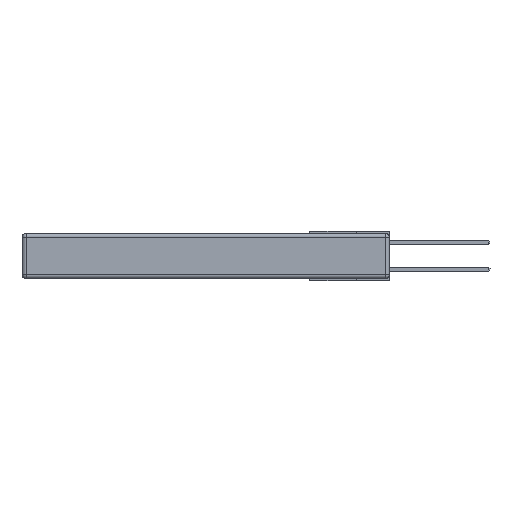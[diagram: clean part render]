
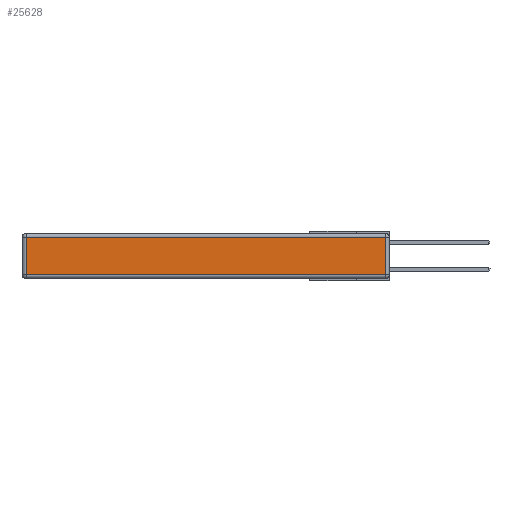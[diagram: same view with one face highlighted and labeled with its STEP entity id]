
A CAD part, left-side view. The second image highlights one B-rep face of the part: STEP entity #25628.
In plain terms, the highlighted planar face has unit normal (-1, 0, 0).
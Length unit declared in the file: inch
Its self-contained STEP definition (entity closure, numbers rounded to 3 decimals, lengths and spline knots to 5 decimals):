
#993 = VERTEX_POINT ( 'NONE', #25898 ) ;
#1000 = CARTESIAN_POINT ( 'NONE',  ( 0., 0.03, -0.03 ) ) ;
#3266 = VECTOR ( 'NONE', #28624, 39.37008 ) ;
#3453 = EDGE_CURVE ( 'NONE', #15135, #5135, #9915, .T. ) ;
#4842 = CARTESIAN_POINT ( 'NONE',  ( 0., 0.03, -0.343 ) ) ;
#5065 = LINE ( 'NONE', #4842, #3266 ) ;
#5135 = VERTEX_POINT ( 'NONE', #28177 ) ;
#7178 = ORIENTED_EDGE ( 'NONE', *, *, #8831, .T. ) ;
#7296 = DIRECTION ( 'NONE',  ( 0., -1., 0. ) ) ;
#8421 = ORIENTED_EDGE ( 'NONE', *, *, #14954, .T. ) ;
#8831 = EDGE_CURVE ( 'NONE', #13798, #993, #24177, .T. ) ;
#9138 = AXIS2_PLACEMENT_3D ( 'NONE', #18822, #28046, #21138 ) ;
#9915 = LINE ( 'NONE', #20629, #15360 ) ;
#10405 = ORIENTED_EDGE ( 'NONE', *, *, #3453, .T. ) ;
#10896 = CARTESIAN_POINT ( 'NONE',  ( 0., 2.72, -0.313 ) ) ;
#12630 = CARTESIAN_POINT ( 'NONE',  ( 0., 2.72, -0.343 ) ) ;
#13610 = PLANE ( 'NONE',  #9138 ) ;
#13798 = VERTEX_POINT ( 'NONE', #10896 ) ;
#13987 = CARTESIAN_POINT ( 'NONE',  ( 0., 0., -0.313 ) ) ;
#14954 = EDGE_CURVE ( 'NONE', #5135, #13798, #27329, .T. ) ;
#15135 = VERTEX_POINT ( 'NONE', #1000 ) ;
#15360 = VECTOR ( 'NONE', #25102, 39.37008 ) ;
#17255 = DIRECTION ( 'NONE',  ( 0., 0., -1. ) ) ;
#18000 = VECTOR ( 'NONE', #7296, 39.37008 ) ;
#18822 = CARTESIAN_POINT ( 'NONE',  ( 0., 0., -0.343 ) ) ;
#19465 = FACE_OUTER_BOUND ( 'NONE', #22830, .T. ) ;
#20629 = CARTESIAN_POINT ( 'NONE',  ( 0., 2.75, -0.03 ) ) ;
#21138 = DIRECTION ( 'NONE',  ( 0., 0., 1. ) ) ;
#21162 = VECTOR ( 'NONE', #17255, 39.37008 ) ;
#22830 = EDGE_LOOP ( 'NONE', ( #7178, #26344, #10405, #8421 ) ) ;
#24177 = LINE ( 'NONE', #13987, #18000 ) ;
#25102 = DIRECTION ( 'NONE',  ( 0., 1., 0. ) ) ;
#25628 = ADVANCED_FACE ( 'NONE', ( #19465 ), #13610, .T. ) ;
#25898 = CARTESIAN_POINT ( 'NONE',  ( 0., 0.03, -0.313 ) ) ;
#26344 = ORIENTED_EDGE ( 'NONE', *, *, #26486, .T. ) ;
#26486 = EDGE_CURVE ( 'NONE', #993, #15135, #5065, .T. ) ;
#27329 = LINE ( 'NONE', #12630, #21162 ) ;
#28046 = DIRECTION ( 'NONE',  ( -1., 0., 0. ) ) ;
#28177 = CARTESIAN_POINT ( 'NONE',  ( 0., 2.72, -0.03 ) ) ;
#28624 = DIRECTION ( 'NONE',  ( 0., 0., 1. ) ) ;
